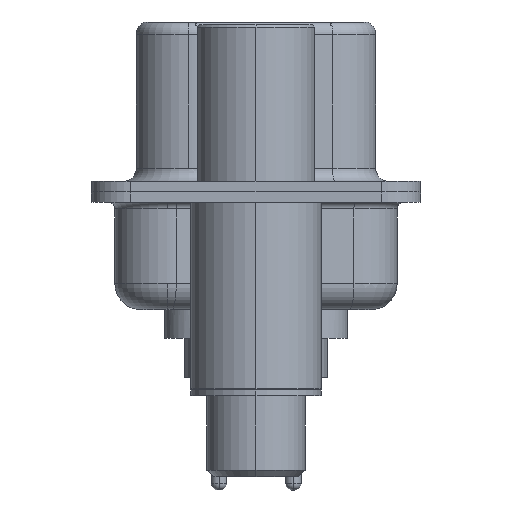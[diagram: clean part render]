
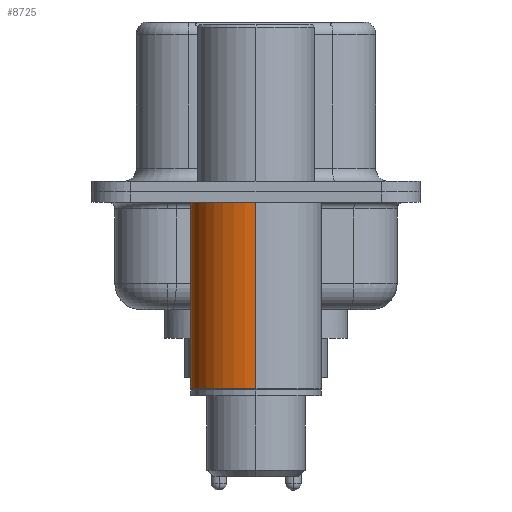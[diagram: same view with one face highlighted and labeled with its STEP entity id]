
A CAD part, left-side view. The second image highlights one B-rep face of the part: STEP entity #8725.
In plain terms, the highlighted cylindrical face has radius 2.5 mm (diameter 5 mm), a partial arc.
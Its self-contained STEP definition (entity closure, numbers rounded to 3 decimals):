
#4005 = DIRECTION ( 'NONE',  ( 0., 0., 1. ) ) ;
#4298 = LINE ( 'NONE', #17970, #9672 ) ;
#4354 = AXIS2_PLACEMENT_3D ( 'NONE', #24923, #11118, #27218 ) ;
#4575 = VERTEX_POINT ( 'NONE', #28134 ) ;
#4877 = CARTESIAN_POINT ( 'NONE',  ( 2.5, 0., 0.581 ) ) ;
#7197 = ORIENTED_EDGE ( 'NONE', *, *, #26094, .T. ) ;
#7992 = EDGE_CURVE ( 'NONE', #18576, #4575, #4298, .T. ) ;
#8291 = VECTOR ( 'NONE', #18668, 1000. ) ;
#8471 = CIRCLE ( 'NONE', #19915, 2.5 ) ;
#8725 = ADVANCED_FACE ( 'NONE', ( #24402 ), #12898, .T. ) ;
#9672 = VECTOR ( 'NONE', #24909, 1000. ) ;
#11118 = DIRECTION ( 'NONE',  ( 0., 0., 1. ) ) ;
#12898 = CYLINDRICAL_SURFACE ( 'NONE', #23336, 2.5 ) ;
#12989 = ORIENTED_EDGE ( 'NONE', *, *, #7992, .T. ) ;
#14288 = VERTEX_POINT ( 'NONE', #20600 ) ;
#15118 = CARTESIAN_POINT ( 'NONE',  ( 2.5, 0., -0.4 ) ) ;
#17786 = CARTESIAN_POINT ( 'NONE',  ( 0., 0., -7.525 ) ) ;
#17970 = CARTESIAN_POINT ( 'NONE',  ( -2.5, 0., 0.581 ) ) ;
#18576 = VERTEX_POINT ( 'NONE', #22051 ) ;
#18603 = VERTEX_POINT ( 'NONE', #15118 ) ;
#18668 = DIRECTION ( 'NONE',  ( 0., 0., 1. ) ) ;
#19390 = EDGE_CURVE ( 'NONE', #18603, #4575, #22234, .T. ) ;
#19915 = AXIS2_PLACEMENT_3D ( 'NONE', #17786, #4005, #20121 ) ;
#20121 = DIRECTION ( 'NONE',  ( 1., 0., 0. ) ) ;
#20165 = DIRECTION ( 'NONE',  ( 1., 0., 0. ) ) ;
#20600 = CARTESIAN_POINT ( 'NONE',  ( 2.5, 0., -7.525 ) ) ;
#22051 = CARTESIAN_POINT ( 'NONE',  ( -2.5, 0., -7.525 ) ) ;
#22234 = CIRCLE ( 'NONE', #4354, 2.5 ) ;
#22445 = CARTESIAN_POINT ( 'NONE',  ( 0., 0., 0.581 ) ) ;
#23336 = AXIS2_PLACEMENT_3D ( 'NONE', #22445, #24739, #20165 ) ;
#24001 = EDGE_LOOP ( 'NONE', ( #7197, #12989, #27268, #26190 ) ) ;
#24402 = FACE_OUTER_BOUND ( 'NONE', #24001, .T. ) ;
#24739 = DIRECTION ( 'NONE',  ( 0., 0., 1. ) ) ;
#24909 = DIRECTION ( 'NONE',  ( 0., 0., 1. ) ) ;
#24923 = CARTESIAN_POINT ( 'NONE',  ( 0., 0., -0.4 ) ) ;
#25908 = LINE ( 'NONE', #4877, #8291 ) ;
#26094 = EDGE_CURVE ( 'NONE', #14288, #18576, #8471, .T. ) ;
#26190 = ORIENTED_EDGE ( 'NONE', *, *, #29546, .F. ) ;
#27218 = DIRECTION ( 'NONE',  ( 1., 0., 0. ) ) ;
#27268 = ORIENTED_EDGE ( 'NONE', *, *, #19390, .F. ) ;
#28134 = CARTESIAN_POINT ( 'NONE',  ( -2.5, 0., -0.4 ) ) ;
#29546 = EDGE_CURVE ( 'NONE', #14288, #18603, #25908, .T. ) ;
